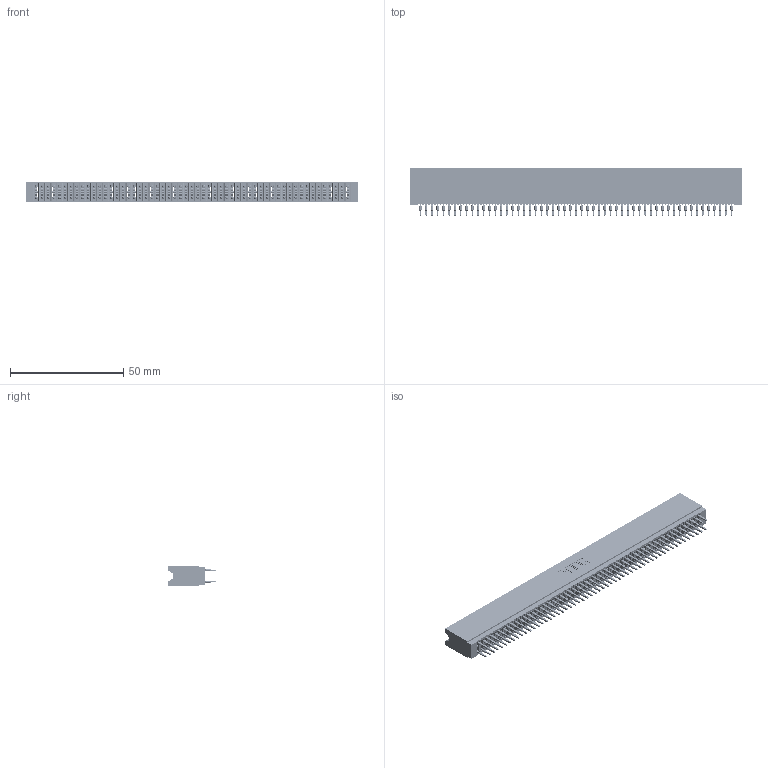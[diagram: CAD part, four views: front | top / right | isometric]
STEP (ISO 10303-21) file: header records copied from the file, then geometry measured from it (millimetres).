
FILE_DESCRIPTION (( 'STEP AP203' ), '1' );
FILE_NAME ('745-110-560-206.STEP', '2026-02-27T00:26:14', ( '' ), ( '' ), 'SwSTEP 2.0', 'SolidWorks 2023', '' );
FILE_SCHEMA (( 'CONFIG_CONTROL_DESIGN' ));
Length unit declared in the file: millimetre
Products named in the file (3): 745-110-560-206; 745-292-001_560; 745 Part_Insulator Option - 06
Assembly tree (111 placements, depth 2):
  745-110-560-206
    745 Part_Insulator Option - 06
    745-292-001_560  x110
Bounding box: 146.3 x 21.22 x 8.89 mm (x, y, z)
Volume: 13481.5 mm3; surface area: 29470.3 mm2
Topology: 111 solids, 111 shells, 10931 faces, 29905 edges, 18982 vertices
Faces by surface type: plane 5666, cylinder 2405, bspline 2200, torus 660
Entity records: 91162 total; most frequent: CARTESIAN_POINT 16312, ORIENTED_EDGE 15774, DIRECTION 13773, EDGE_CURVE 7887, LINE 7367, VECTOR 7367, VERTEX_POINT 5030, AXIS2_PLACEMENT_3D 3203
